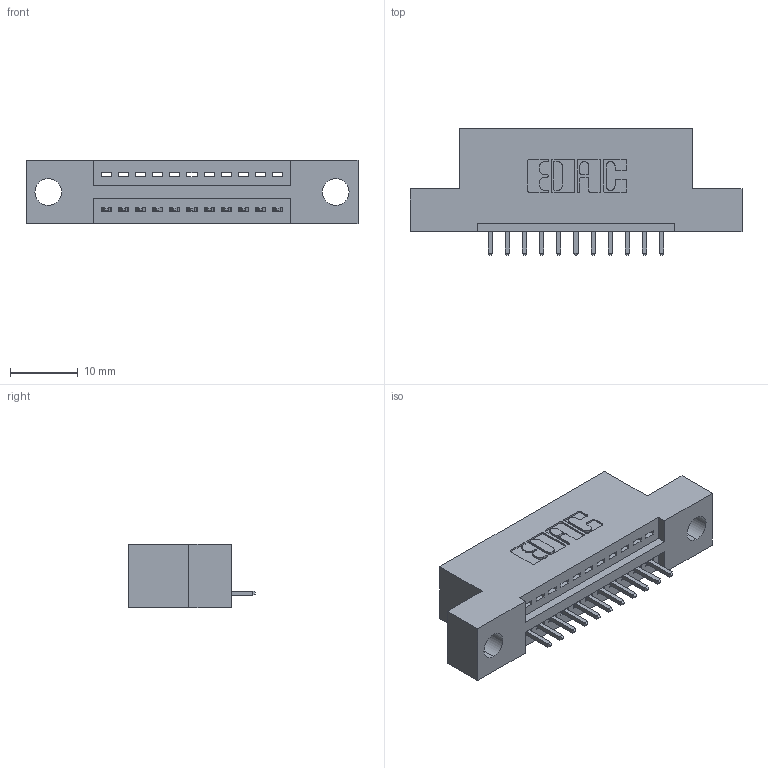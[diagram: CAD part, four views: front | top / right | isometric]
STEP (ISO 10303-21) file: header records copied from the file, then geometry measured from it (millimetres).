
FILE_DESCRIPTION (( 'STEP AP203' ), '1' );
FILE_NAME ('395-011-521-104.STEP', '2021-05-31T14:16:02', ( '' ), ( '' ), 'SwSTEP 2.0', 'SolidWorks 2020', '' );
FILE_SCHEMA (( 'CONFIG_CONTROL_DESIGN' ));
Length unit declared in the file: inch
Products named in the file (3): 345-292-001_345-293-121; 345 Part_Flush Mounting Lugs - 0.156 Dia-TI; 395-011-521-104
Assembly tree (12 placements, depth 2):
  395-011-521-104
    345 Part_Flush Mounting Lugs - 0.156 Dia-TI
    345-292-001_345-293-121  x11
Bounding box: 49.15 x 18.72 x 9.4 mm (x, y, z)
Volume: 4277 mm3; surface area: 4982.5 mm2
Topology: 12 solids, 12 shells, 778 faces, 2313 edges, 1526 vertices
Faces by surface type: plane 534, cylinder 244
Entity records: 12889 total; most frequent: CARTESIAN_POINT 2243, ORIENTED_EDGE 2186, DIRECTION 2003, EDGE_CURVE 1093, LINE 917, VECTOR 917, VERTEX_POINT 726, AXIS2_PLACEMENT_3D 543
